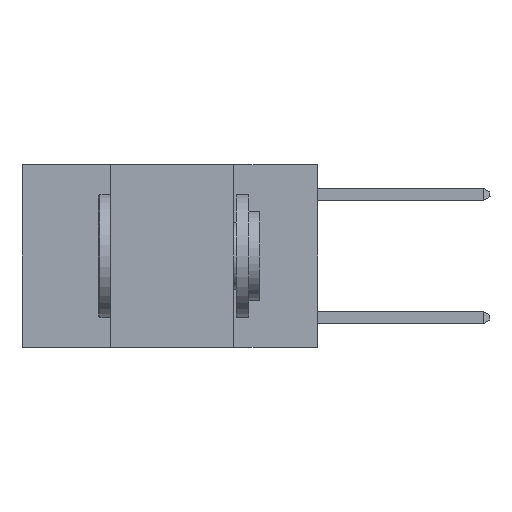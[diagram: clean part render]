
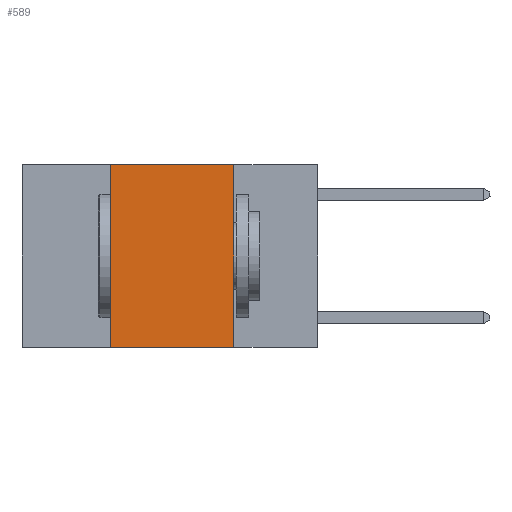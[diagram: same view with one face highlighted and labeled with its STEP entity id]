
A CAD part, left-side view. The second image highlights one B-rep face of the part: STEP entity #589.
In plain terms, the highlighted planar face has unit normal (-1, 0, 0).
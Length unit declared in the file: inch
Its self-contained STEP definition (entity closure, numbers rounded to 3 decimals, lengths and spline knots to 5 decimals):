
#589 = ADVANCED_FACE ( 'NONE', ( #23030 ), #11421, .F. ) ;
#1597 = ORIENTED_EDGE ( 'NONE', *, *, #5255, .F. ) ;
#1906 = CARTESIAN_POINT ( 'NONE',  ( 0., 0.17, 0. ) ) ;
#2552 = LINE ( 'NONE', #23633, #22048 ) ;
#2591 = EDGE_CURVE ( 'NONE', #15410, #9174, #18810, .T. ) ;
#3082 = LINE ( 'NONE', #6801, #9021 ) ;
#4698 = VECTOR ( 'NONE', #17648, 39.37008 ) ;
#5255 = EDGE_CURVE ( 'NONE', #15410, #15063, #3082, .T. ) ;
#5663 = AXIS2_PLACEMENT_3D ( 'NONE', #19119, #17714, #18021 ) ;
#5880 = EDGE_LOOP ( 'NONE', ( #21119, #16698, #1597, #7539 ) ) ;
#6476 = EDGE_CURVE ( 'NONE', #15063, #18838, #2552, .T. ) ;
#6801 = CARTESIAN_POINT ( 'NONE',  ( 0., 0.42, 0. ) ) ;
#6916 = DIRECTION ( 'NONE',  ( 0., -1., 0. ) ) ;
#7539 = ORIENTED_EDGE ( 'NONE', *, *, #2591, .T. ) ;
#9021 = VECTOR ( 'NONE', #22273, 39.37008 ) ;
#9174 = VERTEX_POINT ( 'NONE', #19650 ) ;
#10216 = DIRECTION ( 'NONE',  ( 0., -1., 0. ) ) ;
#10873 = CARTESIAN_POINT ( 'NONE',  ( 0., 0.6, -0.37 ) ) ;
#11421 = PLANE ( 'NONE',  #5663 ) ;
#13176 = EDGE_CURVE ( 'NONE', #18838, #9174, #20242, .T. ) ;
#13352 = CARTESIAN_POINT ( 'NONE',  ( 0., 0.42, 0. ) ) ;
#13689 = VECTOR ( 'NONE', #6916, 39.37008 ) ;
#15063 = VERTEX_POINT ( 'NONE', #13352 ) ;
#15410 = VERTEX_POINT ( 'NONE', #16315 ) ;
#16315 = CARTESIAN_POINT ( 'NONE',  ( 0., 0.42, -0.37 ) ) ;
#16456 = CARTESIAN_POINT ( 'NONE',  ( 0., 0.17, 0. ) ) ;
#16698 = ORIENTED_EDGE ( 'NONE', *, *, #6476, .F. ) ;
#17648 = DIRECTION ( 'NONE',  ( 0., 0., -1. ) ) ;
#17714 = DIRECTION ( 'NONE',  ( 1., 0., 0. ) ) ;
#18021 = DIRECTION ( 'NONE',  ( 0., 0., -1. ) ) ;
#18810 = LINE ( 'NONE', #10873, #13689 ) ;
#18838 = VERTEX_POINT ( 'NONE', #16456 ) ;
#19119 = CARTESIAN_POINT ( 'NONE',  ( 0., 0.6, 0. ) ) ;
#19650 = CARTESIAN_POINT ( 'NONE',  ( 0., 0.17, -0.37 ) ) ;
#20242 = LINE ( 'NONE', #1906, #4698 ) ;
#21119 = ORIENTED_EDGE ( 'NONE', *, *, #13176, .F. ) ;
#22048 = VECTOR ( 'NONE', #10216, 39.37008 ) ;
#22273 = DIRECTION ( 'NONE',  ( 0., 0., 1. ) ) ;
#23030 = FACE_OUTER_BOUND ( 'NONE', #5880, .T. ) ;
#23633 = CARTESIAN_POINT ( 'NONE',  ( 0., 0.6, 0. ) ) ;
